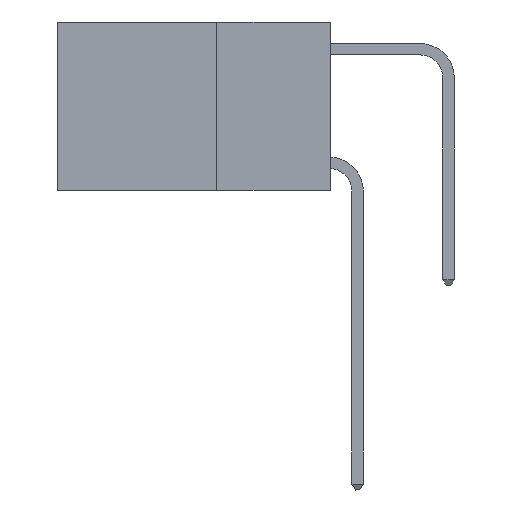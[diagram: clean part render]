
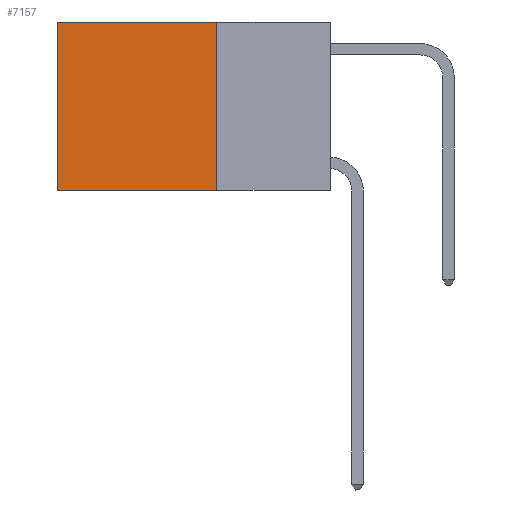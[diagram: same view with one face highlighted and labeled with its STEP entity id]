
A CAD part, left-side view. The second image highlights one B-rep face of the part: STEP entity #7157.
In plain terms, the highlighted planar face has unit normal (-1, 0, 0).
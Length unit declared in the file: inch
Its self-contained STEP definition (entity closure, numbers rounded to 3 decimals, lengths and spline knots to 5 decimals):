
#110 = LINE ( 'NONE', #741, #6778 ) ;
#727 = VERTEX_POINT ( 'NONE', #14588 ) ;
#741 = CARTESIAN_POINT ( 'NONE',  ( 0.2625, 0.25, 0. ) ) ;
#1708 = CARTESIAN_POINT ( 'NONE',  ( 0.2625, 0.25, -0.37 ) ) ;
#2318 = LINE ( 'NONE', #19799, #4140 ) ;
#2880 = DIRECTION ( 'NONE',  ( 1., 0., 0. ) ) ;
#2884 = LINE ( 'NONE', #6201, #8979 ) ;
#3087 = DIRECTION ( 'NONE',  ( 0., 1., 0. ) ) ;
#3540 = EDGE_LOOP ( 'NONE', ( #7695, #12109, #10526, #5009 ) ) ;
#4140 = VECTOR ( 'NONE', #16608, 39.37008 ) ;
#4646 = VERTEX_POINT ( 'NONE', #18730 ) ;
#4837 = VECTOR ( 'NONE', #3087, 39.37008 ) ;
#5009 = ORIENTED_EDGE ( 'NONE', *, *, #5998, .T. ) ;
#5996 = DIRECTION ( 'NONE',  ( 0., 0., -1. ) ) ;
#5998 = EDGE_CURVE ( 'NONE', #17525, #4646, #14373, .T. ) ;
#6201 = CARTESIAN_POINT ( 'NONE',  ( 0.2625, 0.6, 0. ) ) ;
#6778 = VECTOR ( 'NONE', #10237, 39.37008 ) ;
#7157 = ADVANCED_FACE ( 'NONE', ( #18517 ), #12395, .F. ) ;
#7695 = ORIENTED_EDGE ( 'NONE', *, *, #8459, .T. ) ;
#7928 = EDGE_CURVE ( 'NONE', #15115, #727, #2318, .T. ) ;
#8459 = EDGE_CURVE ( 'NONE', #4646, #727, #2884, .T. ) ;
#8979 = VECTOR ( 'NONE', #5996, 39.37008 ) ;
#9873 = CARTESIAN_POINT ( 'NONE',  ( 0.2625, 0.25, 0. ) ) ;
#10134 = EDGE_CURVE ( 'NONE', #17525, #15115, #110, .T. ) ;
#10237 = DIRECTION ( 'NONE',  ( 0., 0., -1. ) ) ;
#10369 = AXIS2_PLACEMENT_3D ( 'NONE', #15496, #2880, #10626 ) ;
#10526 = ORIENTED_EDGE ( 'NONE', *, *, #10134, .F. ) ;
#10626 = DIRECTION ( 'NONE',  ( 0., 0., -1. ) ) ;
#12109 = ORIENTED_EDGE ( 'NONE', *, *, #7928, .F. ) ;
#12395 = PLANE ( 'NONE',  #10369 ) ;
#12823 = CARTESIAN_POINT ( 'NONE',  ( 0.2625, 0.25, 0. ) ) ;
#14373 = LINE ( 'NONE', #12823, #4837 ) ;
#14588 = CARTESIAN_POINT ( 'NONE',  ( 0.2625, 0.6, -0.37 ) ) ;
#15115 = VERTEX_POINT ( 'NONE', #1708 ) ;
#15496 = CARTESIAN_POINT ( 'NONE',  ( 0.2625, 0.25, 0. ) ) ;
#16608 = DIRECTION ( 'NONE',  ( 0., 1., 0. ) ) ;
#17525 = VERTEX_POINT ( 'NONE', #9873 ) ;
#18517 = FACE_OUTER_BOUND ( 'NONE', #3540, .T. ) ;
#18730 = CARTESIAN_POINT ( 'NONE',  ( 0.2625, 0.6, 0. ) ) ;
#19799 = CARTESIAN_POINT ( 'NONE',  ( 0.2625, 0.25, -0.37 ) ) ;
